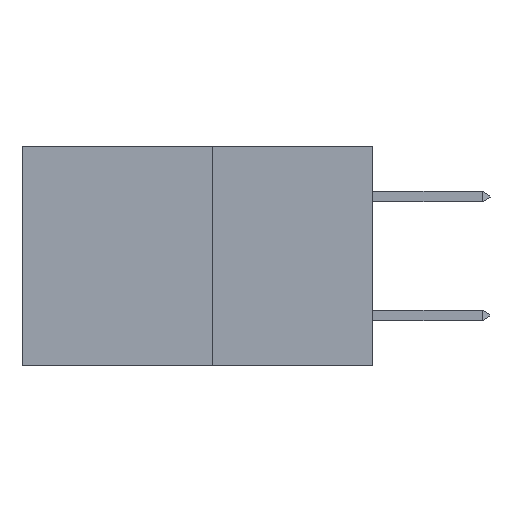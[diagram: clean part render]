
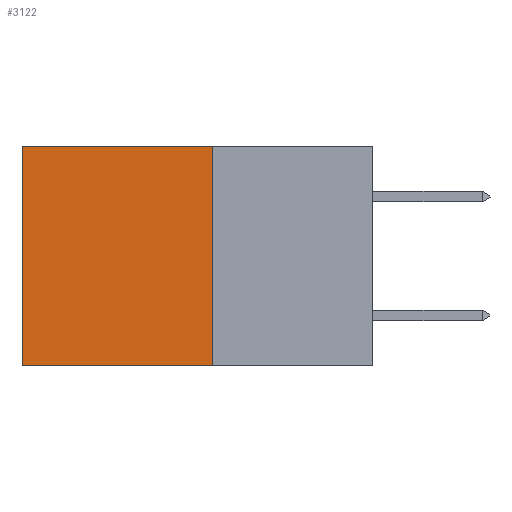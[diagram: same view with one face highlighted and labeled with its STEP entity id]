
A CAD part, left-side view. The second image highlights one B-rep face of the part: STEP entity #3122.
In plain terms, the highlighted planar face has unit normal (-1, 0, 0).
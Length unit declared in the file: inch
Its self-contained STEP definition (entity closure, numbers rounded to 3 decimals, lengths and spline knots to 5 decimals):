
#652 = CARTESIAN_POINT ( 'NONE',  ( 0.277, 0.27, -0.37 ) ) ;
#742 = PLANE ( 'NONE',  #11410 ) ;
#911 = FACE_OUTER_BOUND ( 'NONE', #2621, .T. ) ;
#1327 = VECTOR ( 'NONE', #10206, 39.37008 ) ;
#2126 = VECTOR ( 'NONE', #14613, 39.37008 ) ;
#2621 = EDGE_LOOP ( 'NONE', ( #13949, #15018, #9644, #13062 ) ) ;
#2692 = CARTESIAN_POINT ( 'NONE',  ( 0.277, 0.27, -0.37 ) ) ;
#3122 = ADVANCED_FACE ( 'NONE', ( #911 ), #742, .F. ) ;
#3558 = VECTOR ( 'NONE', #7894, 39.37008 ) ;
#4359 = VERTEX_POINT ( 'NONE', #13200 ) ;
#4859 = VERTEX_POINT ( 'NONE', #7828 ) ;
#6368 = CARTESIAN_POINT ( 'NONE',  ( 0.277, 0.59, 0. ) ) ;
#7150 = LINE ( 'NONE', #2692, #9837 ) ;
#7344 = LINE ( 'NONE', #12517, #1327 ) ;
#7828 = CARTESIAN_POINT ( 'NONE',  ( 0.277, 0.59, -0.37 ) ) ;
#7890 = CARTESIAN_POINT ( 'NONE',  ( 0.277, 0.27, 0. ) ) ;
#7894 = DIRECTION ( 'NONE',  ( 0., 1., 0. ) ) ;
#8182 = DIRECTION ( 'NONE',  ( 0., 0., -1. ) ) ;
#9644 = ORIENTED_EDGE ( 'NONE', *, *, #15135, .F. ) ;
#9837 = VECTOR ( 'NONE', #10872, 39.37008 ) ;
#10004 = VERTEX_POINT ( 'NONE', #11665 ) ;
#10112 = EDGE_CURVE ( 'NONE', #4359, #4859, #7150, .T. ) ;
#10206 = DIRECTION ( 'NONE',  ( 0., 0., -1. ) ) ;
#10558 = EDGE_CURVE ( 'NONE', #10004, #12086, #12860, .T. ) ;
#10872 = DIRECTION ( 'NONE',  ( 0., 1., 0. ) ) ;
#11410 = AXIS2_PLACEMENT_3D ( 'NONE', #652, #14821, #8182 ) ;
#11665 = CARTESIAN_POINT ( 'NONE',  ( 0.277, 0.27, 0. ) ) ;
#12086 = VERTEX_POINT ( 'NONE', #6368 ) ;
#12517 = CARTESIAN_POINT ( 'NONE',  ( 0.277, 0.27, -0.37 ) ) ;
#12860 = LINE ( 'NONE', #7890, #3558 ) ;
#12973 = EDGE_CURVE ( 'NONE', #12086, #4859, #14187, .T. ) ;
#13062 = ORIENTED_EDGE ( 'NONE', *, *, #10558, .T. ) ;
#13200 = CARTESIAN_POINT ( 'NONE',  ( 0.277, 0.27, -0.37 ) ) ;
#13477 = CARTESIAN_POINT ( 'NONE',  ( 0.277, 0.59, -0.37 ) ) ;
#13949 = ORIENTED_EDGE ( 'NONE', *, *, #12973, .T. ) ;
#14187 = LINE ( 'NONE', #13477, #2126 ) ;
#14613 = DIRECTION ( 'NONE',  ( 0., 0., -1. ) ) ;
#14821 = DIRECTION ( 'NONE',  ( 1., 0., 0. ) ) ;
#15018 = ORIENTED_EDGE ( 'NONE', *, *, #10112, .F. ) ;
#15135 = EDGE_CURVE ( 'NONE', #10004, #4359, #7344, .T. ) ;
